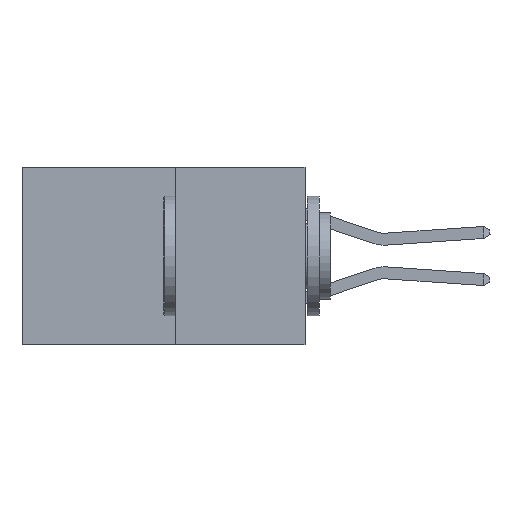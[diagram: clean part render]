
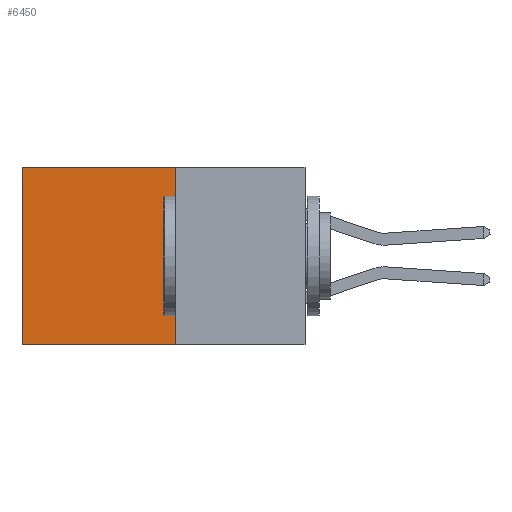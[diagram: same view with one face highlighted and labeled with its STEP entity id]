
A CAD part, left-side view. The second image highlights one B-rep face of the part: STEP entity #6450.
In plain terms, the highlighted planar face has unit normal (-1, 0, 0).
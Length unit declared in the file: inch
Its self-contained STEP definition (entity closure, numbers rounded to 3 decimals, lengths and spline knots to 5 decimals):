
#405 = CARTESIAN_POINT ( 'NONE',  ( 0.277, 0.59, -0.37 ) ) ;
#457 = CARTESIAN_POINT ( 'NONE',  ( 0.277, 0.27, 0. ) ) ;
#485 = DIRECTION ( 'NONE',  ( 0., 1., 0. ) ) ;
#546 = CARTESIAN_POINT ( 'NONE',  ( 0.277, 0.27, -0.37 ) ) ;
#1256 = ORIENTED_EDGE ( 'NONE', *, *, #5584, .F. ) ;
#1265 = CARTESIAN_POINT ( 'NONE',  ( 0.277, 0.27, -0.37 ) ) ;
#1566 = DIRECTION ( 'NONE',  ( 0., 0., -1. ) ) ;
#2231 = FACE_OUTER_BOUND ( 'NONE', #3574, .T. ) ;
#2607 = EDGE_CURVE ( 'NONE', #8130, #3536, #3675, .T. ) ;
#2808 = ORIENTED_EDGE ( 'NONE', *, *, #3999, .F. ) ;
#2979 = VERTEX_POINT ( 'NONE', #546 ) ;
#3536 = VERTEX_POINT ( 'NONE', #9205 ) ;
#3574 = EDGE_LOOP ( 'NONE', ( #9040, #1256, #2808, #7011 ) ) ;
#3675 = LINE ( 'NONE', #457, #5867 ) ;
#3751 = AXIS2_PLACEMENT_3D ( 'NONE', #4417, #4333, #4307 ) ;
#3885 = VECTOR ( 'NONE', #5281, 39.37008 ) ;
#3999 = EDGE_CURVE ( 'NONE', #8130, #2979, #4144, .T. ) ;
#4144 = LINE ( 'NONE', #1265, #6340 ) ;
#4307 = DIRECTION ( 'NONE',  ( 0., 0., -1. ) ) ;
#4333 = DIRECTION ( 'NONE',  ( 1., 0., 0. ) ) ;
#4338 = LINE ( 'NONE', #5850, #8275 ) ;
#4417 = CARTESIAN_POINT ( 'NONE',  ( 0.277, 0.27, -0.37 ) ) ;
#4437 = PLANE ( 'NONE',  #3751 ) ;
#5281 = DIRECTION ( 'NONE',  ( 0., 1., 0. ) ) ;
#5475 = CARTESIAN_POINT ( 'NONE',  ( 0.277, 0.27, -0.37 ) ) ;
#5502 = DIRECTION ( 'NONE',  ( 0., 0., -1. ) ) ;
#5574 = EDGE_CURVE ( 'NONE', #3536, #6740, #4338, .T. ) ;
#5584 = EDGE_CURVE ( 'NONE', #2979, #6740, #5857, .T. ) ;
#5850 = CARTESIAN_POINT ( 'NONE',  ( 0.277, 0.59, -0.37 ) ) ;
#5857 = LINE ( 'NONE', #5475, #3885 ) ;
#5867 = VECTOR ( 'NONE', #485, 39.37008 ) ;
#6340 = VECTOR ( 'NONE', #1566, 39.37008 ) ;
#6450 = ADVANCED_FACE ( 'NONE', ( #2231 ), #4437, .F. ) ;
#6740 = VERTEX_POINT ( 'NONE', #405 ) ;
#6835 = CARTESIAN_POINT ( 'NONE',  ( 0.277, 0.27, 0. ) ) ;
#7011 = ORIENTED_EDGE ( 'NONE', *, *, #2607, .T. ) ;
#8130 = VERTEX_POINT ( 'NONE', #6835 ) ;
#8275 = VECTOR ( 'NONE', #5502, 39.37008 ) ;
#9040 = ORIENTED_EDGE ( 'NONE', *, *, #5574, .T. ) ;
#9205 = CARTESIAN_POINT ( 'NONE',  ( 0.277, 0.59, 0. ) ) ;
